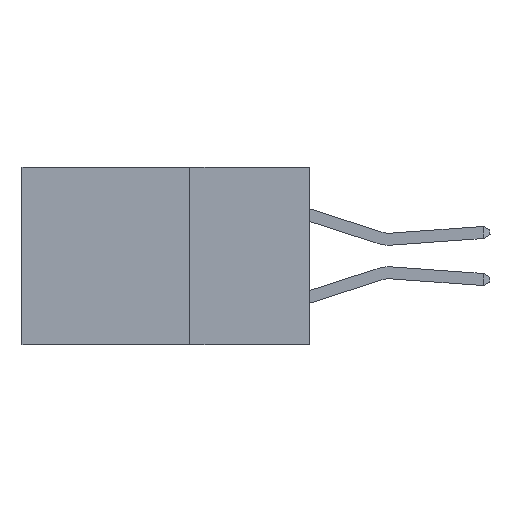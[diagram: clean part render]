
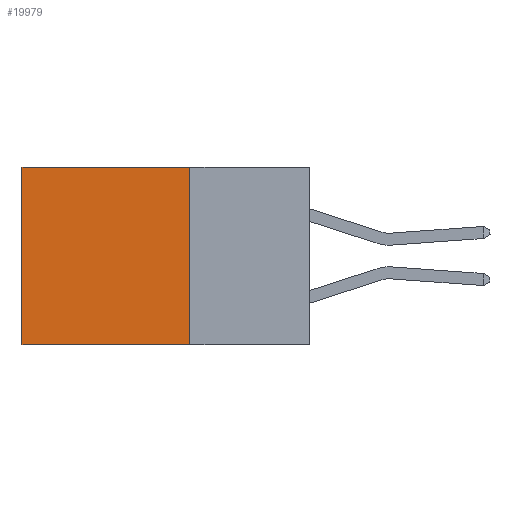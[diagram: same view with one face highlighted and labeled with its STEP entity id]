
A CAD part, left-side view. The second image highlights one B-rep face of the part: STEP entity #19979.
In plain terms, the highlighted planar face has unit normal (-1, 0, 0).
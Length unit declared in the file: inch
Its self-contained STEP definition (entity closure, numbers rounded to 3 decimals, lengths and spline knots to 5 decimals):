
#919 = CARTESIAN_POINT ( 'NONE',  ( 0.2615, 0.25, -0.37 ) ) ;
#972 = ORIENTED_EDGE ( 'NONE', *, *, #15230, .F. ) ;
#1121 = DIRECTION ( 'NONE',  ( 1., 0., 0. ) ) ;
#1401 = DIRECTION ( 'NONE',  ( 0., 0., -1. ) ) ;
#1426 = DIRECTION ( 'NONE',  ( 0., 1., 0. ) ) ;
#1998 = CARTESIAN_POINT ( 'NONE',  ( 0.2615, 0.6, -0.37 ) ) ;
#2470 = CARTESIAN_POINT ( 'NONE',  ( 0.2615, 0.25, 0. ) ) ;
#3039 = LINE ( 'NONE', #20569, #12041 ) ;
#3613 = EDGE_CURVE ( 'NONE', #15831, #9504, #12666, .T. ) ;
#4009 = PLANE ( 'NONE',  #5167 ) ;
#4222 = ORIENTED_EDGE ( 'NONE', *, *, #3613, .T. ) ;
#5167 = AXIS2_PLACEMENT_3D ( 'NONE', #919, #1121, #5816 ) ;
#5816 = DIRECTION ( 'NONE',  ( 0., 0., -1. ) ) ;
#5885 = EDGE_CURVE ( 'NONE', #20447, #18265, #20494, .T. ) ;
#5973 = DIRECTION ( 'NONE',  ( 0., 0., -1. ) ) ;
#5989 = VECTOR ( 'NONE', #5973, 39.37008 ) ;
#6721 = LINE ( 'NONE', #16347, #19136 ) ;
#7303 = CARTESIAN_POINT ( 'NONE',  ( 0.2615, 0.6, 0. ) ) ;
#8313 = DIRECTION ( 'NONE',  ( 0., 1., 0. ) ) ;
#9504 = VERTEX_POINT ( 'NONE', #1998 ) ;
#9602 = CARTESIAN_POINT ( 'NONE',  ( 0.2615, 0.6, -0.37 ) ) ;
#12041 = VECTOR ( 'NONE', #1426, 39.37008 ) ;
#12632 = EDGE_CURVE ( 'NONE', #20447, #15831, #3039, .T. ) ;
#12666 = LINE ( 'NONE', #9602, #14677 ) ;
#14226 = CARTESIAN_POINT ( 'NONE',  ( 0.2615, 0.25, -0.37 ) ) ;
#14677 = VECTOR ( 'NONE', #1401, 39.37008 ) ;
#15101 = ORIENTED_EDGE ( 'NONE', *, *, #5885, .F. ) ;
#15230 = EDGE_CURVE ( 'NONE', #18265, #9504, #6721, .T. ) ;
#15831 = VERTEX_POINT ( 'NONE', #7303 ) ;
#16347 = CARTESIAN_POINT ( 'NONE',  ( 0.2615, 0.25, -0.37 ) ) ;
#16969 = CARTESIAN_POINT ( 'NONE',  ( 0.2615, 0.25, -0.37 ) ) ;
#18069 = EDGE_LOOP ( 'NONE', ( #4222, #972, #15101, #19967 ) ) ;
#18265 = VERTEX_POINT ( 'NONE', #16969 ) ;
#18964 = FACE_OUTER_BOUND ( 'NONE', #18069, .T. ) ;
#19136 = VECTOR ( 'NONE', #8313, 39.37008 ) ;
#19967 = ORIENTED_EDGE ( 'NONE', *, *, #12632, .T. ) ;
#19979 = ADVANCED_FACE ( 'NONE', ( #18964 ), #4009, .F. ) ;
#20447 = VERTEX_POINT ( 'NONE', #2470 ) ;
#20494 = LINE ( 'NONE', #14226, #5989 ) ;
#20569 = CARTESIAN_POINT ( 'NONE',  ( 0.2615, 0.25, 0. ) ) ;
